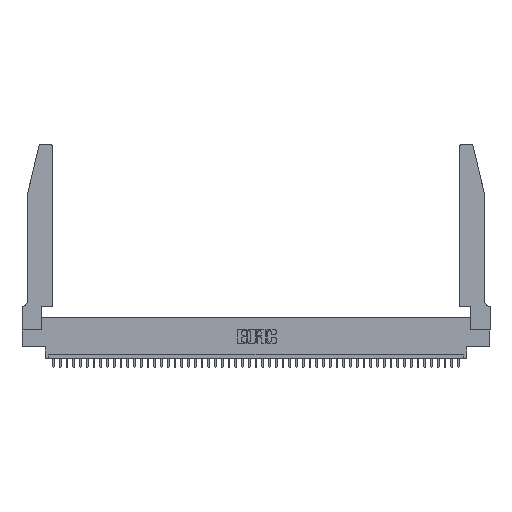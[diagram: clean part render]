
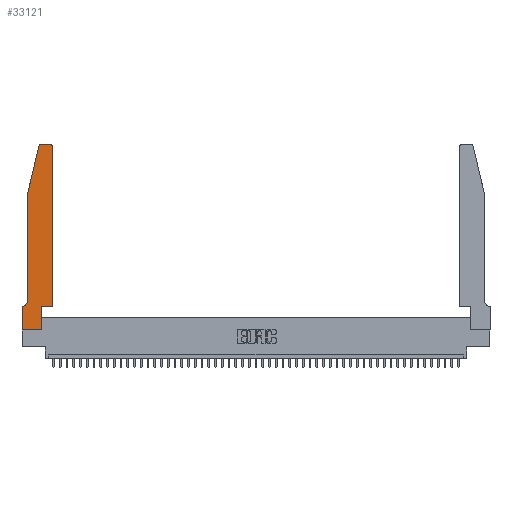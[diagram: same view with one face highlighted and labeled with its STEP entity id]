
A CAD part, top view. The second image highlights one B-rep face of the part: STEP entity #33121.
In plain terms, the highlighted planar face has unit normal (0, 0, 1).
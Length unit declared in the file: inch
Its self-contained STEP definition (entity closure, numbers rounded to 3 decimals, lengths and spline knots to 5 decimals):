
#112 = CARTESIAN_POINT ( 'NONE',  ( 0.25487, 2.72718, 0.37 ) ) ;
#676 = EDGE_CURVE ( 'NONE', #10508, #29292, #22089, .T. ) ;
#689 = ORIENTED_EDGE ( 'NONE', *, *, #8223, .T. ) ;
#1291 = VECTOR ( 'NONE', #8765, 39.37008 ) ;
#1442 = EDGE_CURVE ( 'NONE', #46114, #20834, #30124, .T. ) ;
#1871 = EDGE_CURVE ( 'NONE', #9255, #47167, #14979, .T. ) ;
#2247 = VECTOR ( 'NONE', #32911, 39.37008 ) ;
#2332 = LINE ( 'NONE', #26951, #26193 ) ;
#2379 = CARTESIAN_POINT ( 'NONE',  ( 0.284, 2.72, 0.37 ) ) ;
#2383 = ORIENTED_EDGE ( 'NONE', *, *, #23427, .T. ) ;
#3313 = CARTESIAN_POINT ( 'NONE',  ( 0.0755, 0.42, 0.37 ) ) ;
#3646 = CARTESIAN_POINT ( 'NONE',  ( 0.0055, 0.42, 0.37 ) ) ;
#4033 = CARTESIAN_POINT ( 'NONE',  ( 0.4505, 0.35, 0.37 ) ) ;
#4251 = CARTESIAN_POINT ( 'NONE',  ( 0.284, 2.75, 0.37 ) ) ;
#4460 = AXIS2_PLACEMENT_3D ( 'NONE', #20142, #17373, #17548 ) ;
#5289 = VECTOR ( 'NONE', #27607, 39.37008 ) ;
#5443 = ORIENTED_EDGE ( 'NONE', *, *, #39898, .T. ) ;
#5964 = CARTESIAN_POINT ( 'NONE',  ( 0., 0., 0.37 ) ) ;
#6201 = CARTESIAN_POINT ( 'NONE',  ( 0.0055, 0.35, 0.37 ) ) ;
#6830 = AXIS2_PLACEMENT_3D ( 'NONE', #3646, #10309, #40823 ) ;
#7486 = CARTESIAN_POINT ( 'NONE',  ( 0.4205, 2.72, 0.37 ) ) ;
#7766 = ORIENTED_EDGE ( 'NONE', *, *, #1871, .T. ) ;
#8027 = DIRECTION ( 'NONE',  ( -1., 0., 0. ) ) ;
#8223 = EDGE_CURVE ( 'NONE', #13125, #38282, #21923, .T. ) ;
#8488 = ORIENTED_EDGE ( 'NONE', *, *, #27823, .T. ) ;
#8765 = DIRECTION ( 'NONE',  ( 0., -1., 0. ) ) ;
#9255 = VERTEX_POINT ( 'NONE', #22068 ) ;
#9650 = ORIENTED_EDGE ( 'NONE', *, *, #25348, .T. ) ;
#9913 = VECTOR ( 'NONE', #8027, 39.37008 ) ;
#10309 = DIRECTION ( 'NONE',  ( 0., 0., -1. ) ) ;
#10508 = VERTEX_POINT ( 'NONE', #29169 ) ;
#10966 = VECTOR ( 'NONE', #12117, 39.37008 ) ;
#10968 = EDGE_CURVE ( 'NONE', #20240, #46114, #36865, .T. ) ;
#11152 = EDGE_CURVE ( 'NONE', #20834, #17270, #11806, .T. ) ;
#11806 = LINE ( 'NONE', #31079, #13010 ) ;
#12117 = DIRECTION ( 'NONE',  ( 0., 1., 0. ) ) ;
#12235 = LINE ( 'NONE', #30625, #9913 ) ;
#12508 = CARTESIAN_POINT ( 'NONE',  ( 0.0755, 2., 0.37 ) ) ;
#13010 = VECTOR ( 'NONE', #31430, 39.37008 ) ;
#13125 = VERTEX_POINT ( 'NONE', #4251 ) ;
#14825 = DIRECTION ( 'NONE',  ( 1., 0., 0. ) ) ;
#14979 = LINE ( 'NONE', #5964, #19031 ) ;
#16386 = PLANE ( 'NONE',  #4460 ) ;
#17263 = CARTESIAN_POINT ( 'NONE',  ( 0.2865, 0., 0.37 ) ) ;
#17270 = VERTEX_POINT ( 'NONE', #19564 ) ;
#17373 = DIRECTION ( 'NONE',  ( 0., 0., 1. ) ) ;
#17548 = DIRECTION ( 'NONE',  ( 1., 0., 0. ) ) ;
#19031 = VECTOR ( 'NONE', #36546, 39.37008 ) ;
#19564 = CARTESIAN_POINT ( 'NONE',  ( 0., 0.35, 0.37 ) ) ;
#20142 = CARTESIAN_POINT ( 'NONE',  ( 0., 0.35, 0.37 ) ) ;
#20172 = EDGE_LOOP ( 'NONE', ( #2383, #689, #46200, #32287, #36043, #46150, #8488, #7766, #9650, #27254, #21060, #5443 ) ) ;
#20228 = VERTEX_POINT ( 'NONE', #45685 ) ;
#20240 = VERTEX_POINT ( 'NONE', #12508 ) ;
#20834 = VERTEX_POINT ( 'NONE', #6201 ) ;
#20848 = LINE ( 'NONE', #37656, #10966 ) ;
#21060 = ORIENTED_EDGE ( 'NONE', *, *, #24785, .T. ) ;
#21790 = DIRECTION ( 'NONE',  ( 1., 0., 0. ) ) ;
#21923 = CIRCLE ( 'NONE', #30013, 0.03 ) ;
#22068 = CARTESIAN_POINT ( 'NONE',  ( 0., 0., 0.37 ) ) ;
#22089 = LINE ( 'NONE', #22173, #2247 ) ;
#22173 = CARTESIAN_POINT ( 'NONE',  ( 0.4505, 0.35, 0.37 ) ) ;
#22622 = CIRCLE ( 'NONE', #35868, 0.03 ) ;
#22903 = FACE_OUTER_BOUND ( 'NONE', #20172, .T. ) ;
#23427 = EDGE_CURVE ( 'NONE', #20228, #13125, #12235, .T. ) ;
#24785 = EDGE_CURVE ( 'NONE', #29292, #47491, #20848, .T. ) ;
#25348 = EDGE_CURVE ( 'NONE', #47167, #10508, #46081, .T. ) ;
#26193 = VECTOR ( 'NONE', #34444, 39.37008 ) ;
#26951 = CARTESIAN_POINT ( 'NONE',  ( 0.0755, 2., 0.37 ) ) ;
#27254 = ORIENTED_EDGE ( 'NONE', *, *, #676, .T. ) ;
#27607 = DIRECTION ( 'NONE',  ( 0., 1., 0. ) ) ;
#27793 = VECTOR ( 'NONE', #41374, 39.37008 ) ;
#27823 = EDGE_CURVE ( 'NONE', #17270, #9255, #43549, .T. ) ;
#29169 = CARTESIAN_POINT ( 'NONE',  ( 0.2865, 0.35, 0.37 ) ) ;
#29292 = VERTEX_POINT ( 'NONE', #4033 ) ;
#29890 = CARTESIAN_POINT ( 'NONE',  ( 0.4505, 2.72, 0.37 ) ) ;
#30013 = AXIS2_PLACEMENT_3D ( 'NONE', #2379, #44053, #21790 ) ;
#30124 = CIRCLE ( 'NONE', #6830, 0.07 ) ;
#30625 = CARTESIAN_POINT ( 'NONE',  ( 0.2605, 2.75, 0.37 ) ) ;
#31079 = CARTESIAN_POINT ( 'NONE',  ( 0.0755, 0.35, 0.37 ) ) ;
#31430 = DIRECTION ( 'NONE',  ( -1., 0., 0. ) ) ;
#32287 = ORIENTED_EDGE ( 'NONE', *, *, #10968, .T. ) ;
#32911 = DIRECTION ( 'NONE',  ( 1., 0., 0. ) ) ;
#33121 = ADVANCED_FACE ( 'NONE', ( #22903 ), #16386, .T. ) ;
#34444 = DIRECTION ( 'NONE',  ( -0.239, -0.971, 0. ) ) ;
#35674 = EDGE_CURVE ( 'NONE', #38282, #20240, #2332, .T. ) ;
#35868 = AXIS2_PLACEMENT_3D ( 'NONE', #7486, #37380, #14825 ) ;
#36043 = ORIENTED_EDGE ( 'NONE', *, *, #1442, .T. ) ;
#36546 = DIRECTION ( 'NONE',  ( 1., 0., 0. ) ) ;
#36865 = LINE ( 'NONE', #43964, #1291 ) ;
#37380 = DIRECTION ( 'NONE',  ( 0., 0., 1. ) ) ;
#37656 = CARTESIAN_POINT ( 'NONE',  ( 0.4505, 0.35, 0.37 ) ) ;
#38282 = VERTEX_POINT ( 'NONE', #112 ) ;
#39451 = CARTESIAN_POINT ( 'NONE',  ( 0.2865, 0.35, 0.37 ) ) ;
#39898 = EDGE_CURVE ( 'NONE', #47491, #20228, #22622, .T. ) ;
#40823 = DIRECTION ( 'NONE',  ( -1., 0., 0. ) ) ;
#41374 = DIRECTION ( 'NONE',  ( 0., -1., 0. ) ) ;
#43549 = LINE ( 'NONE', #44192, #27793 ) ;
#43964 = CARTESIAN_POINT ( 'NONE',  ( 0.0755, 2., 0.37 ) ) ;
#44053 = DIRECTION ( 'NONE',  ( 0., 0., 1. ) ) ;
#44192 = CARTESIAN_POINT ( 'NONE',  ( 0., 0., 0.37 ) ) ;
#45685 = CARTESIAN_POINT ( 'NONE',  ( 0.4205, 2.75, 0.37 ) ) ;
#46081 = LINE ( 'NONE', #39451, #5289 ) ;
#46114 = VERTEX_POINT ( 'NONE', #3313 ) ;
#46150 = ORIENTED_EDGE ( 'NONE', *, *, #11152, .T. ) ;
#46200 = ORIENTED_EDGE ( 'NONE', *, *, #35674, .T. ) ;
#47167 = VERTEX_POINT ( 'NONE', #17263 ) ;
#47491 = VERTEX_POINT ( 'NONE', #29890 ) ;
